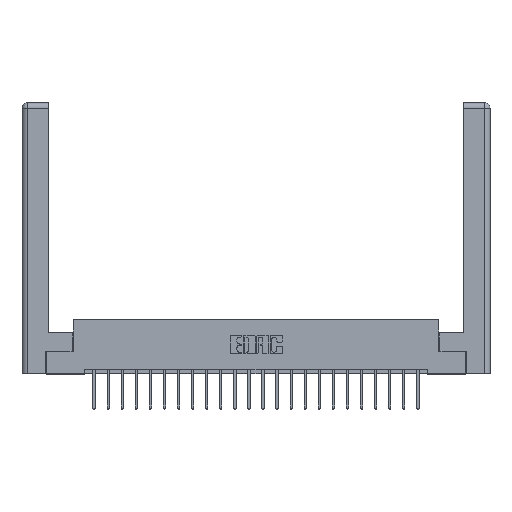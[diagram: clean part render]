
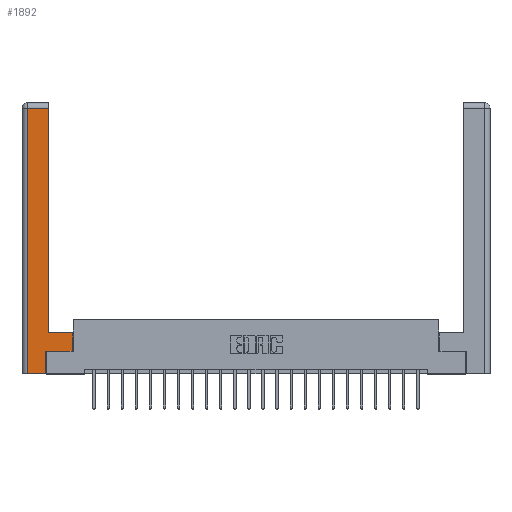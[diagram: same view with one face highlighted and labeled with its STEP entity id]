
A CAD part, top view. The second image highlights one B-rep face of the part: STEP entity #1892.
In plain terms, the highlighted planar face has unit normal (0, 0, 1).
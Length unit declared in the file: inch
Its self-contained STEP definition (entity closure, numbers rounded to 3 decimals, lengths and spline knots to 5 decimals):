
#12 = DIRECTION ( 'NONE',  ( 0., 1., 0. ) ) ;
#418 = VECTOR ( 'NONE', #12, 39.37008 ) ;
#527 = LINE ( 'NONE', #19540, #22756 ) ;
#693 = EDGE_CURVE ( 'NONE', #10003, #21068, #6441, .T. ) ;
#754 = VECTOR ( 'NONE', #3434, 39.37008 ) ;
#1101 = DIRECTION ( 'NONE',  ( -1., 0., 0. ) ) ;
#1513 = ORIENTED_EDGE ( 'NONE', *, *, #17670, .T. ) ;
#1802 = FACE_OUTER_BOUND ( 'NONE', #16683, .T. ) ;
#1892 = ADVANCED_FACE ( 'NONE', ( #1802 ), #14981, .F. ) ;
#2054 = DIRECTION ( 'NONE',  ( 0., 0., -1. ) ) ;
#2258 = AXIS2_PLACEMENT_3D ( 'NONE', #20475, #2054, #18577 ) ;
#2402 = LINE ( 'NONE', #14521, #418 ) ;
#2406 = ORIENTED_EDGE ( 'NONE', *, *, #4505, .T. ) ;
#2673 = LINE ( 'NONE', #4644, #11227 ) ;
#3319 = LINE ( 'NONE', #11137, #21881 ) ;
#3434 = DIRECTION ( 'NONE',  ( 0., 1., 0. ) ) ;
#4505 = EDGE_CURVE ( 'NONE', #6322, #5673, #527, .T. ) ;
#4628 = EDGE_CURVE ( 'NONE', #21330, #10003, #20766, .T. ) ;
#4644 = CARTESIAN_POINT ( 'NONE',  ( 0.0615, 2.94, 0. ) ) ;
#4769 = CARTESIAN_POINT ( 'NONE',  ( 0.295, 0.45, 0. ) ) ;
#4903 = CARTESIAN_POINT ( 'NONE',  ( 0.565, 0.245, 0. ) ) ;
#5673 = VERTEX_POINT ( 'NONE', #12808 ) ;
#5677 = ORIENTED_EDGE ( 'NONE', *, *, #22699, .T. ) ;
#6322 = VERTEX_POINT ( 'NONE', #15993 ) ;
#6441 = LINE ( 'NONE', #14187, #754 ) ;
#6645 = VERTEX_POINT ( 'NONE', #13574 ) ;
#7881 = ORIENTED_EDGE ( 'NONE', *, *, #16054, .T. ) ;
#8009 = CARTESIAN_POINT ( 'NONE',  ( 0.0615, 2.94, 0. ) ) ;
#8078 = CARTESIAN_POINT ( 'NONE',  ( 0.565, 0.245, 0. ) ) ;
#8838 = ORIENTED_EDGE ( 'NONE', *, *, #22487, .T. ) ;
#9205 = DIRECTION ( 'NONE',  ( 0., 1., 0. ) ) ;
#9333 = VECTOR ( 'NONE', #10273, 39.37008 ) ;
#10003 = VERTEX_POINT ( 'NONE', #8078 ) ;
#10273 = DIRECTION ( 'NONE',  ( 1., 0., 0. ) ) ;
#11137 = CARTESIAN_POINT ( 'NONE',  ( 0.265, 0.245, 0. ) ) ;
#11199 = VECTOR ( 'NONE', #1101, 39.37008 ) ;
#11227 = VECTOR ( 'NONE', #13879, 39.37008 ) ;
#11301 = CARTESIAN_POINT ( 'NONE',  ( 0.0615, 0., 0. ) ) ;
#12808 = CARTESIAN_POINT ( 'NONE',  ( 0.265, 0., 0. ) ) ;
#13290 = CARTESIAN_POINT ( 'NONE',  ( 0.565, 0.45, 0. ) ) ;
#13574 = CARTESIAN_POINT ( 'NONE',  ( 0.295, 0.45, 0. ) ) ;
#13879 = DIRECTION ( 'NONE',  ( -1., 0., 0. ) ) ;
#14040 = DIRECTION ( 'NONE',  ( 1., 0., 0. ) ) ;
#14187 = CARTESIAN_POINT ( 'NONE',  ( 0.565, 0.45, 0. ) ) ;
#14521 = CARTESIAN_POINT ( 'NONE',  ( 0.295, 3., 0. ) ) ;
#14981 = PLANE ( 'NONE',  #2258 ) ;
#15216 = CARTESIAN_POINT ( 'NONE',  ( 0.295, 2.94, 0. ) ) ;
#15993 = CARTESIAN_POINT ( 'NONE',  ( 0.0615, 0., 0. ) ) ;
#16037 = LINE ( 'NONE', #4769, #11199 ) ;
#16054 = EDGE_CURVE ( 'NONE', #5673, #21330, #3319, .T. ) ;
#16641 = ORIENTED_EDGE ( 'NONE', *, *, #693, .T. ) ;
#16683 = EDGE_LOOP ( 'NONE', ( #1513, #17008, #8838, #2406, #7881, #18437, #16641, #5677 ) ) ;
#17008 = ORIENTED_EDGE ( 'NONE', *, *, #21922, .T. ) ;
#17670 = EDGE_CURVE ( 'NONE', #6645, #22530, #2402, .T. ) ;
#18147 = VERTEX_POINT ( 'NONE', #8009 ) ;
#18437 = ORIENTED_EDGE ( 'NONE', *, *, #4628, .T. ) ;
#18577 = DIRECTION ( 'NONE',  ( -1., 0., 0. ) ) ;
#18671 = DIRECTION ( 'NONE',  ( 0., -1., 0. ) ) ;
#19540 = CARTESIAN_POINT ( 'NONE',  ( 0.265, 0., 0. ) ) ;
#20475 = CARTESIAN_POINT ( 'NONE',  ( 0., 0., 0. ) ) ;
#20766 = LINE ( 'NONE', #4903, #9333 ) ;
#20893 = VECTOR ( 'NONE', #18671, 39.37008 ) ;
#21068 = VERTEX_POINT ( 'NONE', #13290 ) ;
#21330 = VERTEX_POINT ( 'NONE', #22899 ) ;
#21881 = VECTOR ( 'NONE', #9205, 39.37008 ) ;
#21922 = EDGE_CURVE ( 'NONE', #22530, #18147, #2673, .T. ) ;
#22487 = EDGE_CURVE ( 'NONE', #18147, #6322, #22890, .T. ) ;
#22530 = VERTEX_POINT ( 'NONE', #15216 ) ;
#22699 = EDGE_CURVE ( 'NONE', #21068, #6645, #16037, .T. ) ;
#22756 = VECTOR ( 'NONE', #14040, 39.37008 ) ;
#22890 = LINE ( 'NONE', #11301, #20893 ) ;
#22899 = CARTESIAN_POINT ( 'NONE',  ( 0.265, 0.245, 0. ) ) ;
